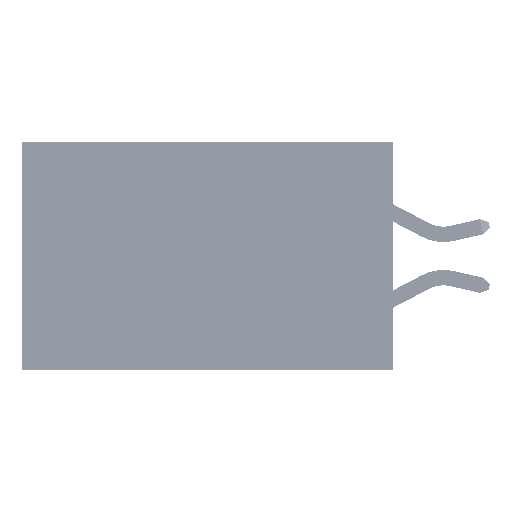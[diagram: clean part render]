
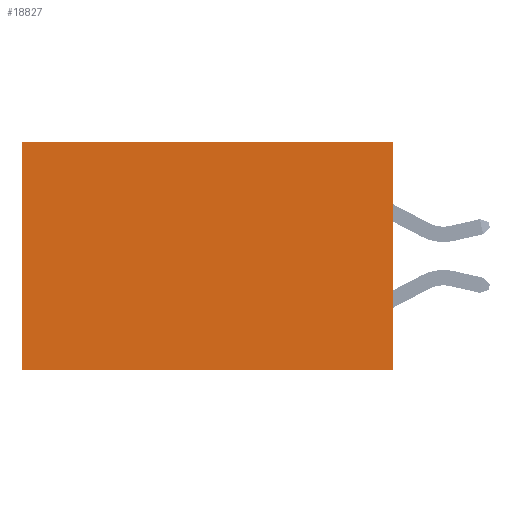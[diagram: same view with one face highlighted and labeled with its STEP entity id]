
A CAD part, left-side view. The second image highlights one B-rep face of the part: STEP entity #18827.
In plain terms, the highlighted planar face has unit normal (-1, 0, 0).
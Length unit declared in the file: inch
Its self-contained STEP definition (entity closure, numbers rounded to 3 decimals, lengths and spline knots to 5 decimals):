
#212 = VECTOR ( 'NONE', #31015, 39.37008 ) ;
#1382 = LINE ( 'NONE', #9631, #212 ) ;
#2747 = EDGE_CURVE ( 'NONE', #7501, #29222, #41318, .T. ) ;
#3108 = EDGE_CURVE ( 'NONE', #45709, #10192, #1382, .T. ) ;
#3110 = VECTOR ( 'NONE', #14166, 39.37008 ) ;
#3275 = EDGE_CURVE ( 'NONE', #7501, #45709, #40152, .T. ) ;
#7501 = VERTEX_POINT ( 'NONE', #40580 ) ;
#9631 = CARTESIAN_POINT ( 'NONE',  ( 0.2875, 0.6, 0. ) ) ;
#10192 = VERTEX_POINT ( 'NONE', #37167 ) ;
#10569 = CARTESIAN_POINT ( 'NONE',  ( 0.2875, 0., 0. ) ) ;
#13378 = DIRECTION ( 'NONE',  ( 0., 0., -1. ) ) ;
#13433 = AXIS2_PLACEMENT_3D ( 'NONE', #31129, #34752, #13378 ) ;
#14166 = DIRECTION ( 'NONE',  ( 0., 1., 0. ) ) ;
#14932 = DIRECTION ( 'NONE',  ( 0., 1., 0. ) ) ;
#14992 = CARTESIAN_POINT ( 'NONE',  ( 0.2875, 0., 0. ) ) ;
#18775 = ORIENTED_EDGE ( 'NONE', *, *, #3275, .T. ) ;
#18827 = ADVANCED_FACE ( 'NONE', ( #42339 ), #27540, .F. ) ;
#21738 = ORIENTED_EDGE ( 'NONE', *, *, #29363, .F. ) ;
#21786 = VECTOR ( 'NONE', #14932, 39.37008 ) ;
#22191 = DIRECTION ( 'NONE',  ( 0., 0., -1. ) ) ;
#27540 = PLANE ( 'NONE',  #13433 ) ;
#28225 = CARTESIAN_POINT ( 'NONE',  ( 0.2875, 0.6, 0. ) ) ;
#29222 = VERTEX_POINT ( 'NONE', #34093 ) ;
#29363 = EDGE_CURVE ( 'NONE', #29222, #10192, #30119, .T. ) ;
#29504 = EDGE_LOOP ( 'NONE', ( #43122, #21738, #33741, #18775 ) ) ;
#30119 = LINE ( 'NONE', #36319, #21786 ) ;
#31015 = DIRECTION ( 'NONE',  ( 0., 0., -1. ) ) ;
#31129 = CARTESIAN_POINT ( 'NONE',  ( 0.2875, 0., 0. ) ) ;
#32855 = VECTOR ( 'NONE', #22191, 39.37008 ) ;
#33741 = ORIENTED_EDGE ( 'NONE', *, *, #2747, .F. ) ;
#34093 = CARTESIAN_POINT ( 'NONE',  ( 0.2875, 0., -0.37 ) ) ;
#34752 = DIRECTION ( 'NONE',  ( 1., 0., 0. ) ) ;
#36319 = CARTESIAN_POINT ( 'NONE',  ( 0.2875, 0., -0.37 ) ) ;
#37167 = CARTESIAN_POINT ( 'NONE',  ( 0.2875, 0.6, -0.37 ) ) ;
#40152 = LINE ( 'NONE', #10569, #3110 ) ;
#40580 = CARTESIAN_POINT ( 'NONE',  ( 0.2875, 0., 0. ) ) ;
#41318 = LINE ( 'NONE', #14992, #32855 ) ;
#42339 = FACE_OUTER_BOUND ( 'NONE', #29504, .T. ) ;
#43122 = ORIENTED_EDGE ( 'NONE', *, *, #3108, .T. ) ;
#45709 = VERTEX_POINT ( 'NONE', #28225 ) ;
